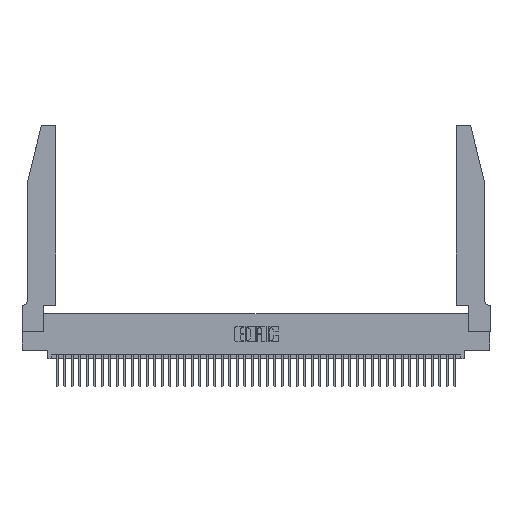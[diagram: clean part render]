
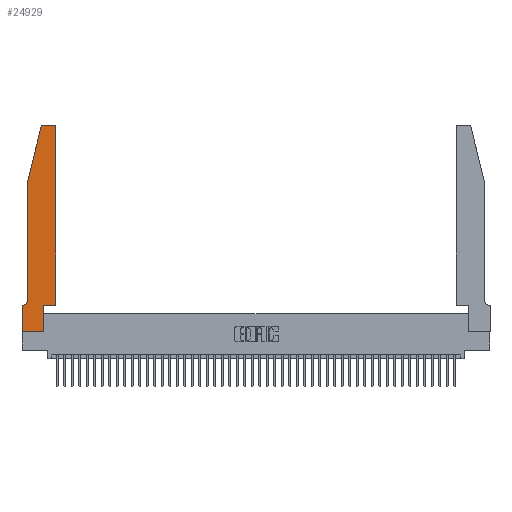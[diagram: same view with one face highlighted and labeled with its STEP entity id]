
A CAD part, top view. The second image highlights one B-rep face of the part: STEP entity #24929.
In plain terms, the highlighted planar face has unit normal (0, 0, 1).
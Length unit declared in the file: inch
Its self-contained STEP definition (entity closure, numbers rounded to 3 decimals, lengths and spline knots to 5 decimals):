
#131 = ORIENTED_EDGE ( 'NONE', *, *, #322, .T. ) ;
#322 = EDGE_CURVE ( 'NONE', #16136, #4608, #22574, .T. ) ;
#593 = VERTEX_POINT ( 'NONE', #13244 ) ;
#2646 = VECTOR ( 'NONE', #4169, 39.37008 ) ;
#3341 = CARTESIAN_POINT ( 'NONE',  ( 0., 0., 0.37 ) ) ;
#3993 = VECTOR ( 'NONE', #27499, 39.37008 ) ;
#4007 = ORIENTED_EDGE ( 'NONE', *, *, #36722, .T. ) ;
#4050 = ORIENTED_EDGE ( 'NONE', *, *, #16002, .T. ) ;
#4169 = DIRECTION ( 'NONE',  ( 0., -1., 0. ) ) ;
#4432 = AXIS2_PLACEMENT_3D ( 'NONE', #27005, #34264, #13136 ) ;
#4608 = VERTEX_POINT ( 'NONE', #38761 ) ;
#4613 = VERTEX_POINT ( 'NONE', #10679 ) ;
#4785 = DIRECTION ( 'NONE',  ( 1., 0., 0. ) ) ;
#5569 = EDGE_CURVE ( 'NONE', #16706, #33475, #31947, .T. ) ;
#5625 = CIRCLE ( 'NONE', #28143, 0.03 ) ;
#5858 = VERTEX_POINT ( 'NONE', #45069 ) ;
#6569 = VERTEX_POINT ( 'NONE', #29810 ) ;
#7392 = ORIENTED_EDGE ( 'NONE', *, *, #43561, .T. ) ;
#7678 = CARTESIAN_POINT ( 'NONE',  ( 0.4205, 2.72, 0.37 ) ) ;
#9088 = DIRECTION ( 'NONE',  ( 0., 0., 1. ) ) ;
#9099 = ORIENTED_EDGE ( 'NONE', *, *, #11371, .T. ) ;
#9534 = PLANE ( 'NONE',  #4432 ) ;
#9818 = VECTOR ( 'NONE', #41268, 39.37008 ) ;
#10679 = CARTESIAN_POINT ( 'NONE',  ( 0.4505, 0.35, 0.37 ) ) ;
#11272 = DIRECTION ( 'NONE',  ( 0., 0., 1. ) ) ;
#11371 = EDGE_CURVE ( 'NONE', #30759, #11995, #39416, .T. ) ;
#11995 = VERTEX_POINT ( 'NONE', #41091 ) ;
#12075 = VECTOR ( 'NONE', #19040, 39.37008 ) ;
#13136 = DIRECTION ( 'NONE',  ( 1., 0., 0. ) ) ;
#13244 = CARTESIAN_POINT ( 'NONE',  ( 0., 0., 0.37 ) ) ;
#14557 = DIRECTION ( 'NONE',  ( 1., 0., 0. ) ) ;
#15890 = CARTESIAN_POINT ( 'NONE',  ( 0.4505, 2.72, 0.37 ) ) ;
#16002 = EDGE_CURVE ( 'NONE', #11995, #5858, #21446, .T. ) ;
#16136 = VERTEX_POINT ( 'NONE', #36678 ) ;
#16706 = VERTEX_POINT ( 'NONE', #35065 ) ;
#16887 = DIRECTION ( 'NONE',  ( 0., -1., 0. ) ) ;
#19040 = DIRECTION ( 'NONE',  ( -1., 0., 0. ) ) ;
#19459 = VECTOR ( 'NONE', #4785, 39.37008 ) ;
#19556 = VECTOR ( 'NONE', #37170, 39.37008 ) ;
#19812 = DIRECTION ( 'NONE',  ( 1., 0., 0. ) ) ;
#20044 = EDGE_CURVE ( 'NONE', #33475, #30759, #36864, .T. ) ;
#21005 = ORIENTED_EDGE ( 'NONE', *, *, #22733, .T. ) ;
#21185 = EDGE_CURVE ( 'NONE', #25628, #593, #24120, .T. ) ;
#21223 = LINE ( 'NONE', #35167, #3993 ) ;
#21446 = LINE ( 'NONE', #42802, #2646 ) ;
#21595 = ORIENTED_EDGE ( 'NONE', *, *, #21185, .T. ) ;
#21910 = CARTESIAN_POINT ( 'NONE',  ( 0.4505, 0.35, 0.37 ) ) ;
#22294 = AXIS2_PLACEMENT_3D ( 'NONE', #45576, #27558, #24494 ) ;
#22574 = LINE ( 'NONE', #38205, #9818 ) ;
#22733 = EDGE_CURVE ( 'NONE', #4613, #37570, #21223, .T. ) ;
#23239 = CARTESIAN_POINT ( 'NONE',  ( 0.2605, 2.75, 0.37 ) ) ;
#24043 = CARTESIAN_POINT ( 'NONE',  ( 0., 0.35, 0.37 ) ) ;
#24120 = LINE ( 'NONE', #3341, #31816 ) ;
#24494 = DIRECTION ( 'NONE',  ( -1., 0., 0. ) ) ;
#24645 = FACE_OUTER_BOUND ( 'NONE', #44757, .T. ) ;
#24907 = LINE ( 'NONE', #21910, #42558 ) ;
#24929 = ADVANCED_FACE ( 'NONE', ( #24645 ), #9534, .T. ) ;
#25628 = VERTEX_POINT ( 'NONE', #24043 ) ;
#25958 = CARTESIAN_POINT ( 'NONE',  ( 0., 0., 0.37 ) ) ;
#26663 = ORIENTED_EDGE ( 'NONE', *, *, #5569, .T. ) ;
#27005 = CARTESIAN_POINT ( 'NONE',  ( 0., 0.35, 0.37 ) ) ;
#27120 = LINE ( 'NONE', #25958, #19459 ) ;
#27130 = CARTESIAN_POINT ( 'NONE',  ( 0.0755, 0.35, 0.37 ) ) ;
#27499 = DIRECTION ( 'NONE',  ( 0., 1., 0. ) ) ;
#27558 = DIRECTION ( 'NONE',  ( 0., 0., -1. ) ) ;
#27559 = EDGE_CURVE ( 'NONE', #5858, #6569, #29313, .T. ) ;
#28143 = AXIS2_PLACEMENT_3D ( 'NONE', #7678, #11272, #14557 ) ;
#29313 = CIRCLE ( 'NONE', #22294, 0.07 ) ;
#29810 = CARTESIAN_POINT ( 'NONE',  ( 0.0055, 0.35, 0.37 ) ) ;
#29992 = LINE ( 'NONE', #27130, #19556 ) ;
#30095 = CARTESIAN_POINT ( 'NONE',  ( 0.284, 2.72, 0.37 ) ) ;
#30303 = ORIENTED_EDGE ( 'NONE', *, *, #37318, .T. ) ;
#30759 = VERTEX_POINT ( 'NONE', #44611 ) ;
#30877 = DIRECTION ( 'NONE',  ( -0.239, -0.971, 0. ) ) ;
#31290 = AXIS2_PLACEMENT_3D ( 'NONE', #30095, #9088, #19812 ) ;
#31816 = VECTOR ( 'NONE', #16887, 39.37008 ) ;
#31947 = LINE ( 'NONE', #23239, #12075 ) ;
#32054 = DIRECTION ( 'NONE',  ( 1., 0., 0. ) ) ;
#33475 = VERTEX_POINT ( 'NONE', #37606 ) ;
#33667 = CARTESIAN_POINT ( 'NONE',  ( 0.0755, 2., 0.37 ) ) ;
#34264 = DIRECTION ( 'NONE',  ( 0., 0., 1. ) ) ;
#35065 = CARTESIAN_POINT ( 'NONE',  ( 0.4205, 2.75, 0.37 ) ) ;
#35167 = CARTESIAN_POINT ( 'NONE',  ( 0.4505, 0.35, 0.37 ) ) ;
#36678 = CARTESIAN_POINT ( 'NONE',  ( 0.2865, 0., 0.37 ) ) ;
#36722 = EDGE_CURVE ( 'NONE', #37570, #16706, #5625, .T. ) ;
#36864 = CIRCLE ( 'NONE', #31290, 0.03 ) ;
#37170 = DIRECTION ( 'NONE',  ( -1., 0., 0. ) ) ;
#37318 = EDGE_CURVE ( 'NONE', #4608, #4613, #24907, .T. ) ;
#37570 = VERTEX_POINT ( 'NONE', #15890 ) ;
#37606 = CARTESIAN_POINT ( 'NONE',  ( 0.284, 2.75, 0.37 ) ) ;
#38205 = CARTESIAN_POINT ( 'NONE',  ( 0.2865, 0.35, 0.37 ) ) ;
#38761 = CARTESIAN_POINT ( 'NONE',  ( 0.2865, 0.35, 0.37 ) ) ;
#39416 = LINE ( 'NONE', #33667, #40575 ) ;
#40575 = VECTOR ( 'NONE', #30877, 39.37008 ) ;
#41079 = ORIENTED_EDGE ( 'NONE', *, *, #20044, .T. ) ;
#41091 = CARTESIAN_POINT ( 'NONE',  ( 0.0755, 2., 0.37 ) ) ;
#41268 = DIRECTION ( 'NONE',  ( 0., 1., 0. ) ) ;
#41597 = ORIENTED_EDGE ( 'NONE', *, *, #42008, .T. ) ;
#42008 = EDGE_CURVE ( 'NONE', #593, #16136, #27120, .T. ) ;
#42558 = VECTOR ( 'NONE', #32054, 39.37008 ) ;
#42802 = CARTESIAN_POINT ( 'NONE',  ( 0.0755, 2., 0.37 ) ) ;
#43364 = ORIENTED_EDGE ( 'NONE', *, *, #27559, .T. ) ;
#43561 = EDGE_CURVE ( 'NONE', #6569, #25628, #29992, .T. ) ;
#44611 = CARTESIAN_POINT ( 'NONE',  ( 0.25487, 2.72718, 0.37 ) ) ;
#44757 = EDGE_LOOP ( 'NONE', ( #26663, #41079, #9099, #4050, #43364, #7392, #21595, #41597, #131, #30303, #21005, #4007 ) ) ;
#45069 = CARTESIAN_POINT ( 'NONE',  ( 0.0755, 0.42, 0.37 ) ) ;
#45576 = CARTESIAN_POINT ( 'NONE',  ( 0.0055, 0.42, 0.37 ) ) ;
